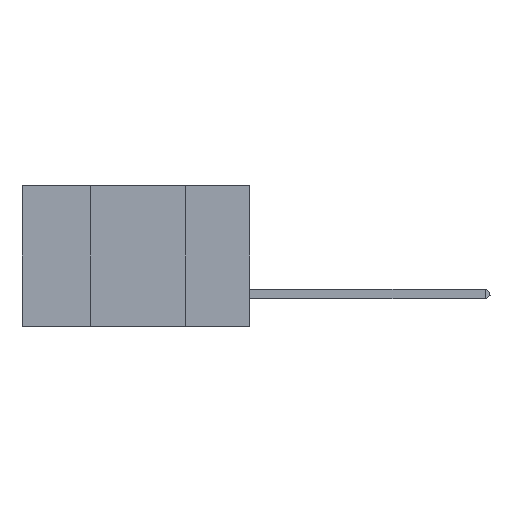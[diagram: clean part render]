
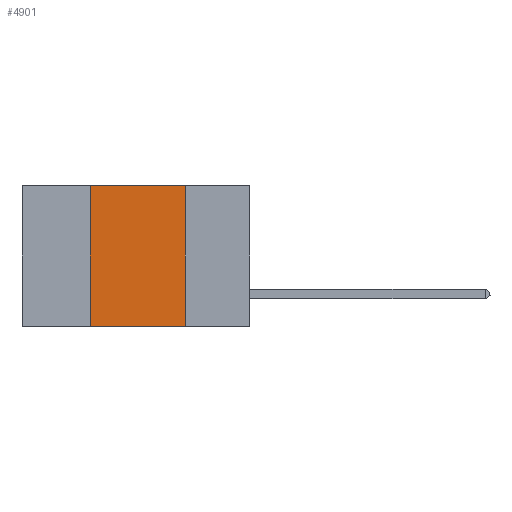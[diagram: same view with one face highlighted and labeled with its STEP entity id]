
A CAD part, left-side view. The second image highlights one B-rep face of the part: STEP entity #4901.
In plain terms, the highlighted planar face has unit normal (-1, 0, 0).
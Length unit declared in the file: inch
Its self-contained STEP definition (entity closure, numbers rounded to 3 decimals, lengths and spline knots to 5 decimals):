
#173 = CARTESIAN_POINT ( 'NONE',  ( 0., 0.17, 0. ) ) ;
#544 = DIRECTION ( 'NONE',  ( 0., -1., 0. ) ) ;
#1472 = LINE ( 'NONE', #22717, #15376 ) ;
#1837 = ORIENTED_EDGE ( 'NONE', *, *, #12573, .T. ) ;
#4538 = CARTESIAN_POINT ( 'NONE',  ( 0., 0.42, 0. ) ) ;
#4901 = ADVANCED_FACE ( 'NONE', ( #22701 ), #20035, .F. ) ;
#6173 = LINE ( 'NONE', #8806, #19638 ) ;
#6515 = CARTESIAN_POINT ( 'NONE',  ( 0., 0.42, -0.37 ) ) ;
#6643 = EDGE_CURVE ( 'NONE', #16730, #21725, #6173, .T. ) ;
#7060 = EDGE_CURVE ( 'NONE', #13683, #19786, #20746, .T. ) ;
#7315 = ORIENTED_EDGE ( 'NONE', *, *, #7060, .F. ) ;
#8554 = DIRECTION ( 'NONE',  ( 0., 0., 1. ) ) ;
#8806 = CARTESIAN_POINT ( 'NONE',  ( 0., 0.42, 0. ) ) ;
#9235 = CARTESIAN_POINT ( 'NONE',  ( 0., 0.6, 0. ) ) ;
#9273 = CARTESIAN_POINT ( 'NONE',  ( 0., 0.17, -0.37 ) ) ;
#9806 = EDGE_LOOP ( 'NONE', ( #7315, #19500, #11709, #1837 ) ) ;
#11709 = ORIENTED_EDGE ( 'NONE', *, *, #6643, .F. ) ;
#12238 = AXIS2_PLACEMENT_3D ( 'NONE', #9235, #14444, #21987 ) ;
#12573 = EDGE_CURVE ( 'NONE', #16730, #19786, #1472, .T. ) ;
#12692 = VECTOR ( 'NONE', #15328, 39.37008 ) ;
#13683 = VERTEX_POINT ( 'NONE', #173 ) ;
#14444 = DIRECTION ( 'NONE',  ( 1., 0., 0. ) ) ;
#14832 = CARTESIAN_POINT ( 'NONE',  ( 0., 0.6, 0. ) ) ;
#15328 = DIRECTION ( 'NONE',  ( 0., 0., -1. ) ) ;
#15376 = VECTOR ( 'NONE', #544, 39.37008 ) ;
#16730 = VERTEX_POINT ( 'NONE', #6515 ) ;
#17195 = VECTOR ( 'NONE', #18554, 39.37008 ) ;
#18554 = DIRECTION ( 'NONE',  ( 0., -1., 0. ) ) ;
#19500 = ORIENTED_EDGE ( 'NONE', *, *, #22110, .F. ) ;
#19638 = VECTOR ( 'NONE', #8554, 39.37008 ) ;
#19786 = VERTEX_POINT ( 'NONE', #9273 ) ;
#20035 = PLANE ( 'NONE',  #12238 ) ;
#20098 = LINE ( 'NONE', #14832, #17195 ) ;
#20746 = LINE ( 'NONE', #21179, #12692 ) ;
#21179 = CARTESIAN_POINT ( 'NONE',  ( 0., 0.17, 0. ) ) ;
#21725 = VERTEX_POINT ( 'NONE', #4538 ) ;
#21987 = DIRECTION ( 'NONE',  ( 0., 0., -1. ) ) ;
#22110 = EDGE_CURVE ( 'NONE', #21725, #13683, #20098, .T. ) ;
#22701 = FACE_OUTER_BOUND ( 'NONE', #9806, .T. ) ;
#22717 = CARTESIAN_POINT ( 'NONE',  ( 0., 0.6, -0.37 ) ) ;
